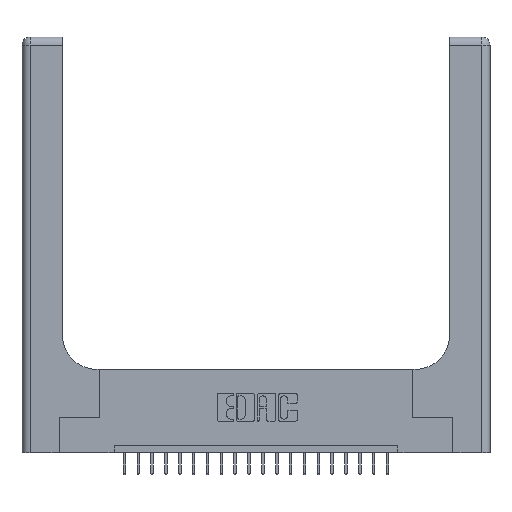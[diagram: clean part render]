
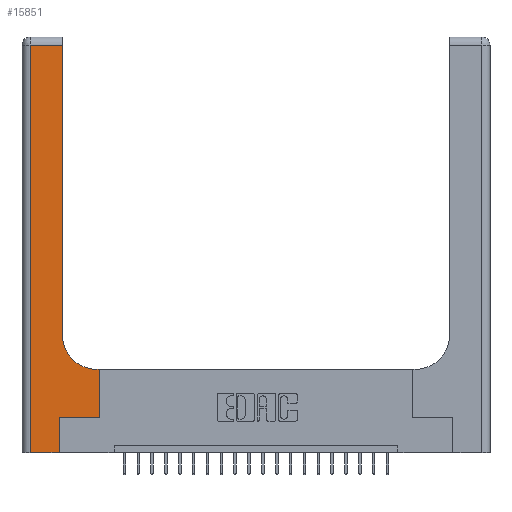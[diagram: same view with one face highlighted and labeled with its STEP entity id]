
A CAD part, top view. The second image highlights one B-rep face of the part: STEP entity #15851.
In plain terms, the highlighted planar face has unit normal (0, 0, 1).
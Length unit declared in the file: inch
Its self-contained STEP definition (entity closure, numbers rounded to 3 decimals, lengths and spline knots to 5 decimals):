
#708 = CARTESIAN_POINT ( 'NONE',  ( 0.5415, 0.6, 0.37 ) ) ;
#1070 = VERTEX_POINT ( 'NONE', #4211 ) ;
#1310 = ORIENTED_EDGE ( 'NONE', *, *, #15437, .T. ) ;
#1503 = VECTOR ( 'NONE', #10331, 39.37008 ) ;
#1690 = EDGE_CURVE ( 'NONE', #1070, #15311, #16427, .T. ) ;
#2026 = CARTESIAN_POINT ( 'NONE',  ( 0.269, 0., 0.37 ) ) ;
#2204 = VECTOR ( 'NONE', #9094, 39.37008 ) ;
#2241 = CARTESIAN_POINT ( 'NONE',  ( 0.06, 3., 0.37 ) ) ;
#2273 = DIRECTION ( 'NONE',  ( -1., 0., 0. ) ) ;
#2492 = DIRECTION ( 'NONE',  ( 0., 1., 0. ) ) ;
#2787 = VERTEX_POINT ( 'NONE', #19879 ) ;
#2991 = VECTOR ( 'NONE', #21092, 39.37008 ) ;
#3343 = VERTEX_POINT ( 'NONE', #10141 ) ;
#3623 = CARTESIAN_POINT ( 'NONE',  ( 0.2915, 0.6, 0.37 ) ) ;
#4211 = CARTESIAN_POINT ( 'NONE',  ( 0.06, 0., 0.37 ) ) ;
#4753 = CARTESIAN_POINT ( 'NONE',  ( 0.269, 0., 0.37 ) ) ;
#4758 = DIRECTION ( 'NONE',  ( -1., 0., 0. ) ) ;
#5042 = VERTEX_POINT ( 'NONE', #9778 ) ;
#5941 = ORIENTED_EDGE ( 'NONE', *, *, #7286, .T. ) ;
#6054 = AXIS2_PLACEMENT_3D ( 'NONE', #21195, #12304, #13776 ) ;
#6877 = LINE ( 'NONE', #2241, #12171 ) ;
#7286 = EDGE_CURVE ( 'NONE', #3343, #1070, #6877, .T. ) ;
#7537 = VERTEX_POINT ( 'NONE', #12399 ) ;
#8400 = AXIS2_PLACEMENT_3D ( 'NONE', #9465, #11090, #2273 ) ;
#8432 = LINE ( 'NONE', #11913, #14003 ) ;
#9094 = DIRECTION ( 'NONE',  ( -1., 0., 0. ) ) ;
#9465 = CARTESIAN_POINT ( 'NONE',  ( 0., 3., 0.37 ) ) ;
#9533 = PLANE ( 'NONE',  #8400 ) ;
#9778 = CARTESIAN_POINT ( 'NONE',  ( 0.5585, 0.6, 0.37 ) ) ;
#10057 = LINE ( 'NONE', #17511, #2991 ) ;
#10133 = EDGE_LOOP ( 'NONE', ( #17939, #1310, #5941, #17668, #17849, #14747, #16975, #18716, #18101 ) ) ;
#10141 = CARTESIAN_POINT ( 'NONE',  ( 0.06, 2.94, 0.37 ) ) ;
#10331 = DIRECTION ( 'NONE',  ( 0., 1., 0. ) ) ;
#10601 = VECTOR ( 'NONE', #17628, 39.37008 ) ;
#10733 = CARTESIAN_POINT ( 'NONE',  ( 0.269, 0.25, 0.37 ) ) ;
#10813 = EDGE_CURVE ( 'NONE', #20969, #7537, #18530, .T. ) ;
#10921 = EDGE_CURVE ( 'NONE', #5042, #20969, #22414, .T. ) ;
#11090 = DIRECTION ( 'NONE',  ( 0., 0., -1. ) ) ;
#11419 = VECTOR ( 'NONE', #2492, 39.37008 ) ;
#11625 = VECTOR ( 'NONE', #15132, 39.37008 ) ;
#11669 = VERTEX_POINT ( 'NONE', #14231 ) ;
#11913 = CARTESIAN_POINT ( 'NONE',  ( 0., 2.94, 0.37 ) ) ;
#11966 = EDGE_CURVE ( 'NONE', #16431, #5042, #10057, .T. ) ;
#12171 = VECTOR ( 'NONE', #16565, 39.37008 ) ;
#12304 = DIRECTION ( 'NONE',  ( 0., 0., -1. ) ) ;
#12399 = CARTESIAN_POINT ( 'NONE',  ( 0.2915, 0.85, 0.37 ) ) ;
#12585 = EDGE_CURVE ( 'NONE', #2787, #16431, #17045, .T. ) ;
#13776 = DIRECTION ( 'NONE',  ( 1., 0., 0. ) ) ;
#14003 = VECTOR ( 'NONE', #4758, 39.37008 ) ;
#14191 = LINE ( 'NONE', #22534, #1503 ) ;
#14231 = CARTESIAN_POINT ( 'NONE',  ( 0.2915, 2.94, 0.37 ) ) ;
#14747 = ORIENTED_EDGE ( 'NONE', *, *, #12585, .T. ) ;
#15132 = DIRECTION ( 'NONE',  ( 1., 0., 0. ) ) ;
#15311 = VERTEX_POINT ( 'NONE', #4753 ) ;
#15437 = EDGE_CURVE ( 'NONE', #11669, #3343, #8432, .T. ) ;
#15851 = ADVANCED_FACE ( 'NONE', ( #20135 ), #9533, .F. ) ;
#15966 = LINE ( 'NONE', #2026, #11419 ) ;
#16427 = LINE ( 'NONE', #20427, #11625 ) ;
#16431 = VERTEX_POINT ( 'NONE', #20674 ) ;
#16565 = DIRECTION ( 'NONE',  ( 0., -1., 0. ) ) ;
#16913 = EDGE_CURVE ( 'NONE', #15311, #2787, #15966, .T. ) ;
#16975 = ORIENTED_EDGE ( 'NONE', *, *, #11966, .T. ) ;
#17045 = LINE ( 'NONE', #10733, #10601 ) ;
#17511 = CARTESIAN_POINT ( 'NONE',  ( 0.5585, 0.25, 0.37 ) ) ;
#17628 = DIRECTION ( 'NONE',  ( 1., 0., 0. ) ) ;
#17668 = ORIENTED_EDGE ( 'NONE', *, *, #1690, .T. ) ;
#17849 = ORIENTED_EDGE ( 'NONE', *, *, #16913, .T. ) ;
#17939 = ORIENTED_EDGE ( 'NONE', *, *, #18100, .T. ) ;
#18100 = EDGE_CURVE ( 'NONE', #7537, #11669, #14191, .T. ) ;
#18101 = ORIENTED_EDGE ( 'NONE', *, *, #10813, .T. ) ;
#18530 = CIRCLE ( 'NONE', #6054, 0.25 ) ;
#18716 = ORIENTED_EDGE ( 'NONE', *, *, #10921, .T. ) ;
#19879 = CARTESIAN_POINT ( 'NONE',  ( 0.269, 0.25, 0.37 ) ) ;
#20135 = FACE_OUTER_BOUND ( 'NONE', #10133, .T. ) ;
#20427 = CARTESIAN_POINT ( 'NONE',  ( 0., 0., 0.37 ) ) ;
#20674 = CARTESIAN_POINT ( 'NONE',  ( 0.5585, 0.25, 0.37 ) ) ;
#20969 = VERTEX_POINT ( 'NONE', #708 ) ;
#21092 = DIRECTION ( 'NONE',  ( 0., 1., 0. ) ) ;
#21195 = CARTESIAN_POINT ( 'NONE',  ( 0.5415, 0.85, 0.37 ) ) ;
#22414 = LINE ( 'NONE', #3623, #2204 ) ;
#22534 = CARTESIAN_POINT ( 'NONE',  ( 0.2915, 3., 0.37 ) ) ;
